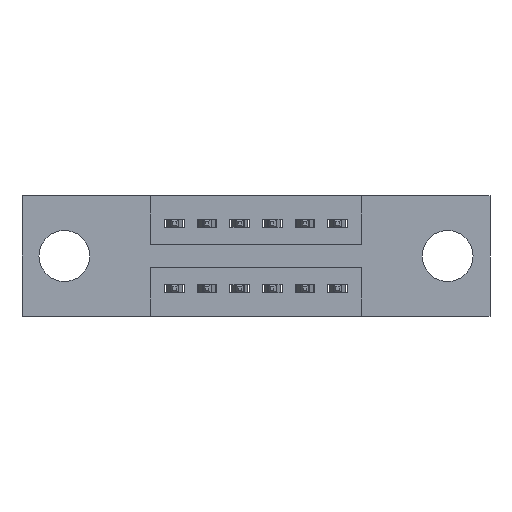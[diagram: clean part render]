
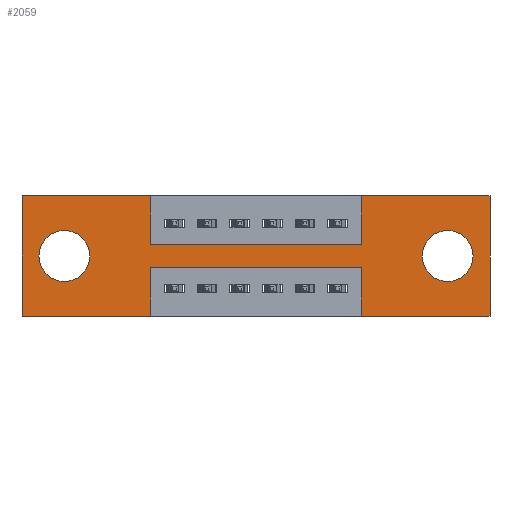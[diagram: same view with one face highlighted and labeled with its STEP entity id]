
A CAD part, front view. The second image highlights one B-rep face of the part: STEP entity #2059.
In plain terms, the highlighted planar face has unit normal (0, -1, 0).
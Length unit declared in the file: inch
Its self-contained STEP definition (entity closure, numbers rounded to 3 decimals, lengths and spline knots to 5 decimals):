
#95 = VECTOR ( 'NONE', #4081, 39.37008 ) ;
#169 = CARTESIAN_POINT ( 'NONE',  ( 0.3925, 0., -0.22 ) ) ;
#236 = DIRECTION ( 'NONE',  ( -1., 0., 0. ) ) ;
#240 = ORIENTED_EDGE ( 'NONE', *, *, #764, .F. ) ;
#294 = EDGE_CURVE ( 'NONE', #2963, #6781, #1192, .T. ) ;
#416 = VECTOR ( 'NONE', #2968, 39.37008 ) ;
#483 = VECTOR ( 'NONE', #4542, 39.37008 ) ;
#516 = FACE_BOUND ( 'NONE', #853, .T. ) ;
#520 = EDGE_CURVE ( 'NONE', #678, #3017, #6357, .T. ) ;
#529 = ORIENTED_EDGE ( 'NONE', *, *, #854, .F. ) ;
#534 = DIRECTION ( 'NONE',  ( 1., 0., 0. ) ) ;
#610 = EDGE_CURVE ( 'NONE', #1280, #1155, #1466, .T. ) ;
#620 = CARTESIAN_POINT ( 'NONE',  ( 1.305, 0., -0.263 ) ) ;
#647 = CARTESIAN_POINT ( 'NONE',  ( 0.3925, 0., -0.15 ) ) ;
#678 = VERTEX_POINT ( 'NONE', #7939 ) ;
#714 = VECTOR ( 'NONE', #5705, 39.37008 ) ;
#719 = DIRECTION ( 'NONE',  ( 0., 0., -1. ) ) ;
#723 = AXIS2_PLACEMENT_3D ( 'NONE', #7028, #9116, #5729 ) ;
#764 = EDGE_CURVE ( 'NONE', #7764, #2963, #8337, .T. ) ;
#853 = EDGE_LOOP ( 'NONE', ( #4133, #6219 ) ) ;
#854 = EDGE_CURVE ( 'NONE', #7916, #7764, #5713, .T. ) ;
#945 = EDGE_CURVE ( 'NONE', #7843, #7916, #3922, .T. ) ;
#952 = DIRECTION ( 'NONE',  ( 0., 0., 1. ) ) ;
#960 = EDGE_CURVE ( 'NONE', #3017, #678, #7419, .T. ) ;
#1025 = EDGE_CURVE ( 'NONE', #2670, #4934, #8126, .T. ) ;
#1155 = VERTEX_POINT ( 'NONE', #8938 ) ;
#1167 = EDGE_CURVE ( 'NONE', #8923, #2670, #2309, .T. ) ;
#1192 = LINE ( 'NONE', #3689, #5087 ) ;
#1280 = VERTEX_POINT ( 'NONE', #7064 ) ;
#1288 = DIRECTION ( 'NONE',  ( 0., 0., -1. ) ) ;
#1329 = EDGE_CURVE ( 'NONE', #6670, #8923, #6119, .T. ) ;
#1339 = EDGE_CURVE ( 'NONE', #2607, #6670, #7515, .T. ) ;
#1357 = CARTESIAN_POINT ( 'NONE',  ( 1.0425, 0., -0.37 ) ) ;
#1441 = DIRECTION ( 'NONE',  ( -1., 0., 0. ) ) ;
#1456 = VECTOR ( 'NONE', #236, 39.37008 ) ;
#1466 = CIRCLE ( 'NONE', #723, 0.078 ) ;
#1546 = LINE ( 'NONE', #4701, #8941 ) ;
#1825 = EDGE_CURVE ( 'NONE', #4998, #7843, #1546, .T. ) ;
#2034 = ORIENTED_EDGE ( 'NONE', *, *, #960, .T. ) ;
#2059 = ADVANCED_FACE ( 'NONE', ( #5034, #516, #6625 ), #3800, .T. ) ;
#2061 = VECTOR ( 'NONE', #4876, 39.37008 ) ;
#2261 = LINE ( 'NONE', #7484, #5976 ) ;
#2309 = LINE ( 'NONE', #647, #9573 ) ;
#2566 = DIRECTION ( 'NONE',  ( -1., 0., 0. ) ) ;
#2607 = VERTEX_POINT ( 'NONE', #5270 ) ;
#2670 = VERTEX_POINT ( 'NONE', #8752 ) ;
#2705 = CARTESIAN_POINT ( 'NONE',  ( 1.0425, 0., 0. ) ) ;
#2786 = EDGE_CURVE ( 'NONE', #3159, #4998, #2261, .T. ) ;
#2963 = VERTEX_POINT ( 'NONE', #3678 ) ;
#2968 = DIRECTION ( 'NONE',  ( 0., 0., 1. ) ) ;
#3017 = VERTEX_POINT ( 'NONE', #620 ) ;
#3023 = ORIENTED_EDGE ( 'NONE', *, *, #1825, .F. ) ;
#3159 = VERTEX_POINT ( 'NONE', #7952 ) ;
#3246 = EDGE_CURVE ( 'NONE', #4934, #3159, #8175, .T. ) ;
#3271 = ORIENTED_EDGE ( 'NONE', *, *, #1025, .F. ) ;
#3473 = EDGE_LOOP ( 'NONE', ( #240, #529, #4814, #3023, #5048, #6847, #3271, #5259, #7507, #6111, #6325, #4943 ) ) ;
#3678 = CARTESIAN_POINT ( 'NONE',  ( 0.3925, 0., -0.37 ) ) ;
#3689 = CARTESIAN_POINT ( 'NONE',  ( 0., 0., -0.37 ) ) ;
#3800 = PLANE ( 'NONE',  #8523 ) ;
#3813 = DIRECTION ( 'NONE',  ( 0., 0., -1. ) ) ;
#3922 = LINE ( 'NONE', #4855, #2061 ) ;
#4081 = DIRECTION ( 'NONE',  ( 1., 0., 0. ) ) ;
#4133 = ORIENTED_EDGE ( 'NONE', *, *, #610, .T. ) ;
#4265 = CARTESIAN_POINT ( 'NONE',  ( 0., 0., 0. ) ) ;
#4314 = EDGE_LOOP ( 'NONE', ( #7606, #2034 ) ) ;
#4384 = DIRECTION ( 'NONE',  ( 0., 0., -1. ) ) ;
#4422 = DIRECTION ( 'NONE',  ( 0., 1., 0. ) ) ;
#4433 = CARTESIAN_POINT ( 'NONE',  ( 1.305, 0., -0.185 ) ) ;
#4436 = CARTESIAN_POINT ( 'NONE',  ( 0., 0., 0. ) ) ;
#4542 = DIRECTION ( 'NONE',  ( 1., 0., 0. ) ) ;
#4622 = CIRCLE ( 'NONE', #9174, 0.078 ) ;
#4701 = CARTESIAN_POINT ( 'NONE',  ( 0., 0., -0.37 ) ) ;
#4814 = ORIENTED_EDGE ( 'NONE', *, *, #945, .F. ) ;
#4855 = CARTESIAN_POINT ( 'NONE',  ( 1.0425, 0., -0.37 ) ) ;
#4876 = DIRECTION ( 'NONE',  ( 0., 0., 1. ) ) ;
#4934 = VERTEX_POINT ( 'NONE', #5291 ) ;
#4943 = ORIENTED_EDGE ( 'NONE', *, *, #294, .F. ) ;
#4944 = CARTESIAN_POINT ( 'NONE',  ( 0., 0., 0. ) ) ;
#4970 = DIRECTION ( 'NONE',  ( 0., 0., -1. ) ) ;
#4998 = VERTEX_POINT ( 'NONE', #8044 ) ;
#5034 = FACE_BOUND ( 'NONE', #4314, .T. ) ;
#5048 = ORIENTED_EDGE ( 'NONE', *, *, #2786, .F. ) ;
#5068 = CARTESIAN_POINT ( 'NONE',  ( 0.3925, 0., 0. ) ) ;
#5087 = VECTOR ( 'NONE', #2566, 39.37008 ) ;
#5170 = CARTESIAN_POINT ( 'NONE',  ( 0., 0., -0.37 ) ) ;
#5177 = CARTESIAN_POINT ( 'NONE',  ( 0., 0., -0.37 ) ) ;
#5259 = ORIENTED_EDGE ( 'NONE', *, *, #1167, .F. ) ;
#5270 = CARTESIAN_POINT ( 'NONE',  ( 0., 0., 0. ) ) ;
#5291 = CARTESIAN_POINT ( 'NONE',  ( 1.0425, 0., 0. ) ) ;
#5578 = DIRECTION ( 'NONE',  ( 0., 1., 0. ) ) ;
#5612 = EDGE_CURVE ( 'NONE', #6781, #2607, #6166, .T. ) ;
#5705 = DIRECTION ( 'NONE',  ( 0., 0., -1. ) ) ;
#5713 = LINE ( 'NONE', #169, #1456 ) ;
#5729 = DIRECTION ( 'NONE',  ( 0., 0., 1. ) ) ;
#5847 = DIRECTION ( 'NONE',  ( 0., 0., 1. ) ) ;
#5976 = VECTOR ( 'NONE', #719, 39.37008 ) ;
#6111 = ORIENTED_EDGE ( 'NONE', *, *, #1339, .F. ) ;
#6119 = LINE ( 'NONE', #5068, #9463 ) ;
#6166 = LINE ( 'NONE', #4436, #9514 ) ;
#6219 = ORIENTED_EDGE ( 'NONE', *, *, #7395, .T. ) ;
#6325 = ORIENTED_EDGE ( 'NONE', *, *, #5612, .F. ) ;
#6357 = CIRCLE ( 'NONE', #8489, 0.078 ) ;
#6625 = FACE_OUTER_BOUND ( 'NONE', #3473, .T. ) ;
#6670 = VERTEX_POINT ( 'NONE', #7136 ) ;
#6781 = VERTEX_POINT ( 'NONE', #5170 ) ;
#6847 = ORIENTED_EDGE ( 'NONE', *, *, #3246, .F. ) ;
#7028 = CARTESIAN_POINT ( 'NONE',  ( 0.13, 0., -0.185 ) ) ;
#7064 = CARTESIAN_POINT ( 'NONE',  ( 0.13, 0., -0.107 ) ) ;
#7136 = CARTESIAN_POINT ( 'NONE',  ( 0.3925, 0., 0. ) ) ;
#7387 = CARTESIAN_POINT ( 'NONE',  ( 0.3925, 0., -0.37 ) ) ;
#7395 = EDGE_CURVE ( 'NONE', #1155, #1280, #4622, .T. ) ;
#7419 = CIRCLE ( 'NONE', #8671, 0.078 ) ;
#7452 = CARTESIAN_POINT ( 'NONE',  ( 0.3925, 0., -0.15 ) ) ;
#7484 = CARTESIAN_POINT ( 'NONE',  ( 1.435, 0., 0. ) ) ;
#7507 = ORIENTED_EDGE ( 'NONE', *, *, #1329, .F. ) ;
#7515 = LINE ( 'NONE', #4265, #95 ) ;
#7606 = ORIENTED_EDGE ( 'NONE', *, *, #520, .T. ) ;
#7682 = DIRECTION ( 'NONE',  ( 0., -1., 0. ) ) ;
#7764 = VERTEX_POINT ( 'NONE', #9185 ) ;
#7843 = VERTEX_POINT ( 'NONE', #1357 ) ;
#7916 = VERTEX_POINT ( 'NONE', #9298 ) ;
#7939 = CARTESIAN_POINT ( 'NONE',  ( 1.305, 0., -0.107 ) ) ;
#7943 = CARTESIAN_POINT ( 'NONE',  ( 1.305, 0., -0.185 ) ) ;
#7952 = CARTESIAN_POINT ( 'NONE',  ( 1.435, 0., 0. ) ) ;
#8044 = CARTESIAN_POINT ( 'NONE',  ( 1.435, 0., -0.37 ) ) ;
#8126 = LINE ( 'NONE', #2705, #416 ) ;
#8175 = LINE ( 'NONE', #4944, #483 ) ;
#8239 = DIRECTION ( 'NONE',  ( 0., 1., 0. ) ) ;
#8337 = LINE ( 'NONE', #7387, #714 ) ;
#8489 = AXIS2_PLACEMENT_3D ( 'NONE', #7943, #8239, #1288 ) ;
#8523 = AXIS2_PLACEMENT_3D ( 'NONE', #5177, #7682, #3813 ) ;
#8671 = AXIS2_PLACEMENT_3D ( 'NONE', #4433, #4422, #4384 ) ;
#8752 = CARTESIAN_POINT ( 'NONE',  ( 1.0425, 0., -0.15 ) ) ;
#8923 = VERTEX_POINT ( 'NONE', #7452 ) ;
#8938 = CARTESIAN_POINT ( 'NONE',  ( 0.13, 0., -0.263 ) ) ;
#8941 = VECTOR ( 'NONE', #1441, 39.37008 ) ;
#9116 = DIRECTION ( 'NONE',  ( 0., 1., 0. ) ) ;
#9174 = AXIS2_PLACEMENT_3D ( 'NONE', #9592, #5578, #952 ) ;
#9185 = CARTESIAN_POINT ( 'NONE',  ( 0.3925, 0., -0.22 ) ) ;
#9298 = CARTESIAN_POINT ( 'NONE',  ( 1.0425, 0., -0.22 ) ) ;
#9463 = VECTOR ( 'NONE', #4970, 39.37008 ) ;
#9514 = VECTOR ( 'NONE', #5847, 39.37008 ) ;
#9573 = VECTOR ( 'NONE', #534, 39.37008 ) ;
#9592 = CARTESIAN_POINT ( 'NONE',  ( 0.13, 0., -0.185 ) ) ;
